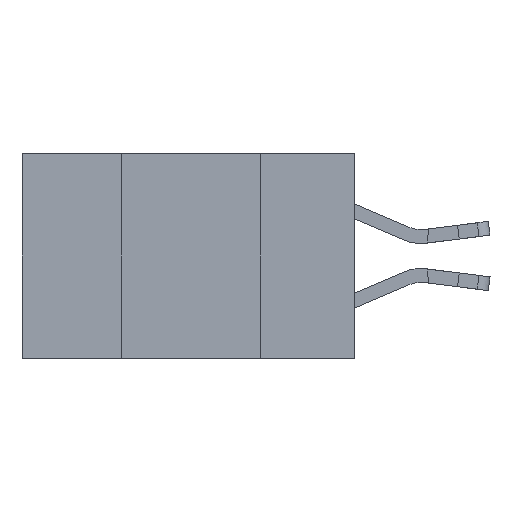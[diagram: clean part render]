
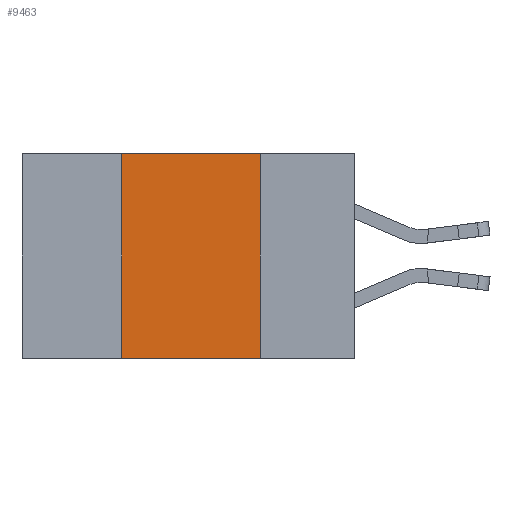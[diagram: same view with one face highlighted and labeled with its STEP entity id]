
A CAD part, left-side view. The second image highlights one B-rep face of the part: STEP entity #9463.
In plain terms, the highlighted planar face has unit normal (-1, 0, 0).
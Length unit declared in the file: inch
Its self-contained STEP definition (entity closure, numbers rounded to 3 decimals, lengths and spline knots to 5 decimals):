
#48 = ORIENTED_EDGE ( 'NONE', *, *, #10098, .F. ) ;
#108 = DIRECTION ( 'NONE',  ( 0., -1., 0. ) ) ;
#472 = VECTOR ( 'NONE', #15405, 39.37008 ) ;
#1452 = VERTEX_POINT ( 'NONE', #16064 ) ;
#1577 = VERTEX_POINT ( 'NONE', #7686 ) ;
#1622 = EDGE_CURVE ( 'NONE', #1452, #1577, #4327, .T. ) ;
#2164 = DIRECTION ( 'NONE',  ( 0., 0., -1. ) ) ;
#2576 = DIRECTION ( 'NONE',  ( 0., 0., 1. ) ) ;
#4327 = LINE ( 'NONE', #6289, #472 ) ;
#5022 = VECTOR ( 'NONE', #2164, 39.37008 ) ;
#6227 = VERTEX_POINT ( 'NONE', #9972 ) ;
#6289 = CARTESIAN_POINT ( 'NONE',  ( 0., 0.6, -0.37 ) ) ;
#6562 = EDGE_CURVE ( 'NONE', #6227, #1577, #11553, .T. ) ;
#6739 = CARTESIAN_POINT ( 'NONE',  ( 0., 0.42, 0. ) ) ;
#7137 = EDGE_LOOP ( 'NONE', ( #7875, #15769, #48, #9853 ) ) ;
#7364 = CARTESIAN_POINT ( 'NONE',  ( 0., 0.6, 0. ) ) ;
#7686 = CARTESIAN_POINT ( 'NONE',  ( 0., 0.17, -0.37 ) ) ;
#7875 = ORIENTED_EDGE ( 'NONE', *, *, #6562, .F. ) ;
#7989 = EDGE_CURVE ( 'NONE', #16503, #6227, #9746, .T. ) ;
#8644 = VECTOR ( 'NONE', #2576, 39.37008 ) ;
#9322 = CARTESIAN_POINT ( 'NONE',  ( 0., 0.6, 0. ) ) ;
#9463 = ADVANCED_FACE ( 'NONE', ( #9700 ), #12566, .F. ) ;
#9700 = FACE_OUTER_BOUND ( 'NONE', #7137, .T. ) ;
#9746 = LINE ( 'NONE', #9322, #12429 ) ;
#9853 = ORIENTED_EDGE ( 'NONE', *, *, #1622, .T. ) ;
#9972 = CARTESIAN_POINT ( 'NONE',  ( 0., 0.17, 0. ) ) ;
#10098 = EDGE_CURVE ( 'NONE', #1452, #16503, #11742, .T. ) ;
#11228 = CARTESIAN_POINT ( 'NONE',  ( 0., 0.17, 0. ) ) ;
#11553 = LINE ( 'NONE', #11228, #5022 ) ;
#11742 = LINE ( 'NONE', #6739, #8644 ) ;
#12429 = VECTOR ( 'NONE', #108, 39.37008 ) ;
#12566 = PLANE ( 'NONE',  #15918 ) ;
#13865 = DIRECTION ( 'NONE',  ( 1., 0., 0. ) ) ;
#14119 = CARTESIAN_POINT ( 'NONE',  ( 0., 0.42, 0. ) ) ;
#15405 = DIRECTION ( 'NONE',  ( 0., -1., 0. ) ) ;
#15769 = ORIENTED_EDGE ( 'NONE', *, *, #7989, .F. ) ;
#15918 = AXIS2_PLACEMENT_3D ( 'NONE', #7364, #13865, #16481 ) ;
#16064 = CARTESIAN_POINT ( 'NONE',  ( 0., 0.42, -0.37 ) ) ;
#16481 = DIRECTION ( 'NONE',  ( 0., 0., -1. ) ) ;
#16503 = VERTEX_POINT ( 'NONE', #14119 ) ;
